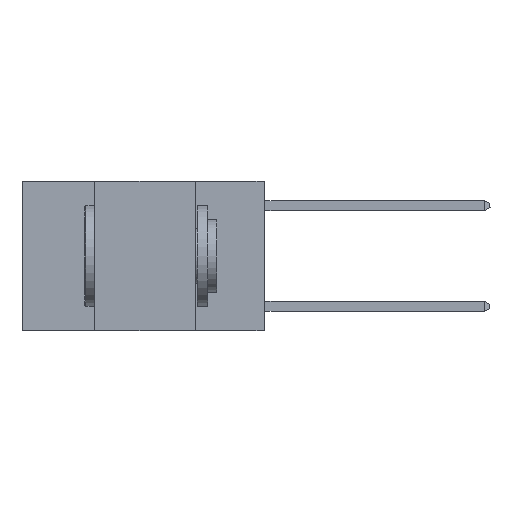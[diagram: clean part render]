
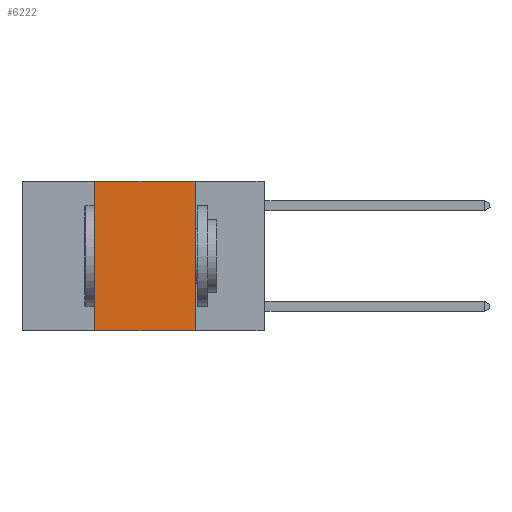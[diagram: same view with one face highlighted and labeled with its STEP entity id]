
A CAD part, left-side view. The second image highlights one B-rep face of the part: STEP entity #6222.
In plain terms, the highlighted planar face has unit normal (-1, 0, 0).
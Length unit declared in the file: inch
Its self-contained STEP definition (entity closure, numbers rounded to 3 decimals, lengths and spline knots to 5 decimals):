
#844 = CARTESIAN_POINT ( 'NONE',  ( 0., 0.6, 0. ) ) ;
#1145 = LINE ( 'NONE', #7750, #11810 ) ;
#1471 = CARTESIAN_POINT ( 'NONE',  ( 0., 0.42, 0. ) ) ;
#2139 = VECTOR ( 'NONE', #6812, 39.37008 ) ;
#2336 = DIRECTION ( 'NONE',  ( 0., 0., -1. ) ) ;
#2868 = VERTEX_POINT ( 'NONE', #13948 ) ;
#3043 = EDGE_CURVE ( 'NONE', #8067, #2868, #16848, .T. ) ;
#3093 = ORIENTED_EDGE ( 'NONE', *, *, #15466, .F. ) ;
#3464 = CARTESIAN_POINT ( 'NONE',  ( 0., 0.17, 0. ) ) ;
#4317 = VERTEX_POINT ( 'NONE', #10873 ) ;
#6206 = VECTOR ( 'NONE', #14467, 39.37008 ) ;
#6222 = ADVANCED_FACE ( 'NONE', ( #16858 ), #16142, .F. ) ;
#6443 = LINE ( 'NONE', #7908, #9715 ) ;
#6555 = VERTEX_POINT ( 'NONE', #3464 ) ;
#6745 = CARTESIAN_POINT ( 'NONE',  ( 0., 0.6, -0.37 ) ) ;
#6812 = DIRECTION ( 'NONE',  ( 0., -1., 0. ) ) ;
#7401 = EDGE_CURVE ( 'NONE', #6555, #2868, #6443, .T. ) ;
#7750 = CARTESIAN_POINT ( 'NONE',  ( 0., 0.6, 0. ) ) ;
#7908 = CARTESIAN_POINT ( 'NONE',  ( 0., 0.17, 0. ) ) ;
#8067 = VERTEX_POINT ( 'NONE', #16390 ) ;
#8976 = ORIENTED_EDGE ( 'NONE', *, *, #16794, .F. ) ;
#9284 = DIRECTION ( 'NONE',  ( 0., 0., -1. ) ) ;
#9715 = VECTOR ( 'NONE', #9284, 39.37008 ) ;
#9923 = LINE ( 'NONE', #1471, #6206 ) ;
#10633 = DIRECTION ( 'NONE',  ( 1., 0., 0. ) ) ;
#10873 = CARTESIAN_POINT ( 'NONE',  ( 0., 0.42, 0. ) ) ;
#11810 = VECTOR ( 'NONE', #14615, 39.37008 ) ;
#12612 = ORIENTED_EDGE ( 'NONE', *, *, #7401, .F. ) ;
#12786 = AXIS2_PLACEMENT_3D ( 'NONE', #844, #10633, #2336 ) ;
#13948 = CARTESIAN_POINT ( 'NONE',  ( 0., 0.17, -0.37 ) ) ;
#14467 = DIRECTION ( 'NONE',  ( 0., 0., 1. ) ) ;
#14615 = DIRECTION ( 'NONE',  ( 0., -1., 0. ) ) ;
#14993 = ORIENTED_EDGE ( 'NONE', *, *, #3043, .T. ) ;
#15466 = EDGE_CURVE ( 'NONE', #8067, #4317, #9923, .T. ) ;
#16142 = PLANE ( 'NONE',  #12786 ) ;
#16390 = CARTESIAN_POINT ( 'NONE',  ( 0., 0.42, -0.37 ) ) ;
#16770 = EDGE_LOOP ( 'NONE', ( #12612, #8976, #3093, #14993 ) ) ;
#16794 = EDGE_CURVE ( 'NONE', #4317, #6555, #1145, .T. ) ;
#16848 = LINE ( 'NONE', #6745, #2139 ) ;
#16858 = FACE_OUTER_BOUND ( 'NONE', #16770, .T. ) ;
